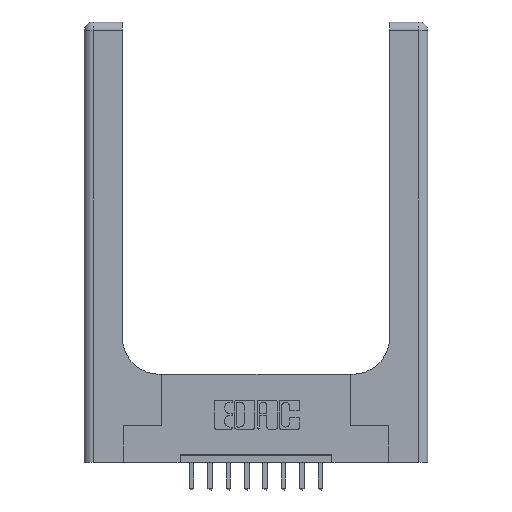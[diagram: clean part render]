
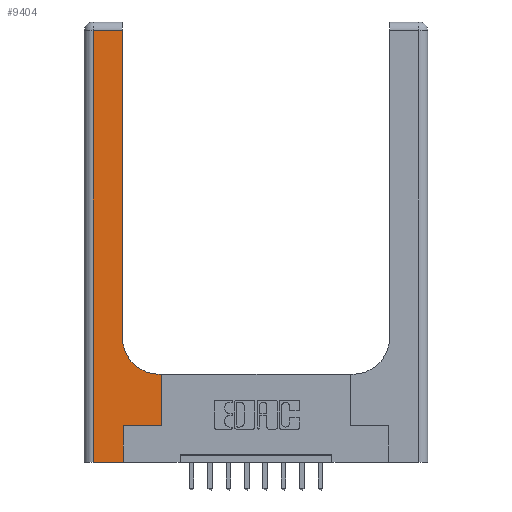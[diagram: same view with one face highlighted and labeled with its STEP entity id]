
A CAD part, top view. The second image highlights one B-rep face of the part: STEP entity #9404.
In plain terms, the highlighted planar face has unit normal (0, 0, 1).
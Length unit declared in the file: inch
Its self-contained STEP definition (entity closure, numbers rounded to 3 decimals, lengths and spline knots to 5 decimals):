
#17 = EDGE_CURVE ( 'NONE', #7598, #47, #6807, .T. ) ;
#47 = VERTEX_POINT ( 'NONE', #12666 ) ;
#351 = EDGE_LOOP ( 'NONE', ( #14441, #14775, #10858, #5102, #4295, #1513, #2029, #2494, #5639 ) ) ;
#426 = VECTOR ( 'NONE', #8383, 39.37008 ) ;
#688 = EDGE_CURVE ( 'NONE', #1045, #2866, #15166, .T. ) ;
#714 = CARTESIAN_POINT ( 'NONE',  ( 0.265, 0.25, 0.37 ) ) ;
#729 = DIRECTION ( 'NONE',  ( -1., 0., 0. ) ) ;
#1045 = VERTEX_POINT ( 'NONE', #714 ) ;
#1513 = ORIENTED_EDGE ( 'NONE', *, *, #688, .T. ) ;
#1601 = EDGE_CURVE ( 'NONE', #14572, #1045, #3699, .T. ) ;
#1659 = CARTESIAN_POINT ( 'NONE',  ( 0.06, 2.94, 0.37 ) ) ;
#1665 = VECTOR ( 'NONE', #5672, 39.37008 ) ;
#2029 = ORIENTED_EDGE ( 'NONE', *, *, #13787, .T. ) ;
#2047 = LINE ( 'NONE', #6753, #11242 ) ;
#2494 = ORIENTED_EDGE ( 'NONE', *, *, #17, .T. ) ;
#2580 = VERTEX_POINT ( 'NONE', #12955 ) ;
#2866 = VERTEX_POINT ( 'NONE', #6545 ) ;
#2950 = CARTESIAN_POINT ( 'NONE',  ( 0.265, 0., 0.37 ) ) ;
#3580 = EDGE_CURVE ( 'NONE', #2580, #14572, #5017, .T. ) ;
#3699 = LINE ( 'NONE', #5850, #426 ) ;
#4295 = ORIENTED_EDGE ( 'NONE', *, *, #1601, .T. ) ;
#4418 = DIRECTION ( 'NONE',  ( 0., 0., -1. ) ) ;
#4563 = DIRECTION ( 'NONE',  ( -1., 0., 0. ) ) ;
#4604 = VECTOR ( 'NONE', #15259, 39.37008 ) ;
#4774 = DIRECTION ( 'NONE',  ( 1., 0., 0. ) ) ;
#4850 = VERTEX_POINT ( 'NONE', #1659 ) ;
#5017 = LINE ( 'NONE', #6262, #9149 ) ;
#5102 = ORIENTED_EDGE ( 'NONE', *, *, #3580, .T. ) ;
#5385 = DIRECTION ( 'NONE',  ( 0., 1., 0. ) ) ;
#5576 = DIRECTION ( 'NONE',  ( 1., 0., 0. ) ) ;
#5639 = ORIENTED_EDGE ( 'NONE', *, *, #14768, .T. ) ;
#5672 = DIRECTION ( 'NONE',  ( 0., 1., 0. ) ) ;
#5713 = PLANE ( 'NONE',  #10213 ) ;
#5850 = CARTESIAN_POINT ( 'NONE',  ( 0.265, 0., 0.37 ) ) ;
#6116 = VECTOR ( 'NONE', #5385, 39.37008 ) ;
#6262 = CARTESIAN_POINT ( 'NONE',  ( 0., 0., 0.37 ) ) ;
#6458 = CARTESIAN_POINT ( 'NONE',  ( 0.26, 0.85, 0.37 ) ) ;
#6545 = CARTESIAN_POINT ( 'NONE',  ( 0.528, 0.25, 0.37 ) ) ;
#6553 = CARTESIAN_POINT ( 'NONE',  ( 0.26, 3., 0.37 ) ) ;
#6753 = CARTESIAN_POINT ( 'NONE',  ( 0., 2.94, 0.37 ) ) ;
#6780 = LINE ( 'NONE', #6553, #6116 ) ;
#6807 = LINE ( 'NONE', #9025, #13244 ) ;
#6991 = LINE ( 'NONE', #11694, #4604 ) ;
#7102 = CARTESIAN_POINT ( 'NONE',  ( 0.51, 0.85, 0.37 ) ) ;
#7260 = VECTOR ( 'NONE', #5576, 39.37008 ) ;
#7598 = VERTEX_POINT ( 'NONE', #15268 ) ;
#7969 = CARTESIAN_POINT ( 'NONE',  ( 0.265, 0.25, 0.37 ) ) ;
#8383 = DIRECTION ( 'NONE',  ( 0., 1., 0. ) ) ;
#9025 = CARTESIAN_POINT ( 'NONE',  ( 0.26, 0.6, 0.37 ) ) ;
#9057 = CARTESIAN_POINT ( 'NONE',  ( 0.26, 2.94, 0.37 ) ) ;
#9149 = VECTOR ( 'NONE', #12057, 39.37008 ) ;
#9404 = ADVANCED_FACE ( 'NONE', ( #15011 ), #5713, .F. ) ;
#9562 = AXIS2_PLACEMENT_3D ( 'NONE', #7102, #14204, #4774 ) ;
#10213 = AXIS2_PLACEMENT_3D ( 'NONE', #14934, #4418, #4563 ) ;
#10307 = EDGE_CURVE ( 'NONE', #12914, #4850, #2047, .T. ) ;
#10858 = ORIENTED_EDGE ( 'NONE', *, *, #13148, .T. ) ;
#11242 = VECTOR ( 'NONE', #729, 39.37008 ) ;
#11694 = CARTESIAN_POINT ( 'NONE',  ( 0.06, 3., 0.37 ) ) ;
#12057 = DIRECTION ( 'NONE',  ( 1., 0., 0. ) ) ;
#12637 = EDGE_CURVE ( 'NONE', #12993, #12914, #6780, .T. ) ;
#12666 = CARTESIAN_POINT ( 'NONE',  ( 0.51, 0.6, 0.37 ) ) ;
#12740 = DIRECTION ( 'NONE',  ( -1., 0., 0. ) ) ;
#12914 = VERTEX_POINT ( 'NONE', #9057 ) ;
#12955 = CARTESIAN_POINT ( 'NONE',  ( 0.06, 0., 0.37 ) ) ;
#12993 = VERTEX_POINT ( 'NONE', #6458 ) ;
#13148 = EDGE_CURVE ( 'NONE', #4850, #2580, #6991, .T. ) ;
#13244 = VECTOR ( 'NONE', #12740, 39.37008 ) ;
#13721 = CARTESIAN_POINT ( 'NONE',  ( 0.528, 0.25, 0.37 ) ) ;
#13787 = EDGE_CURVE ( 'NONE', #2866, #7598, #15039, .T. ) ;
#14204 = DIRECTION ( 'NONE',  ( 0., 0., -1. ) ) ;
#14441 = ORIENTED_EDGE ( 'NONE', *, *, #12637, .T. ) ;
#14501 = CIRCLE ( 'NONE', #9562, 0.25 ) ;
#14572 = VERTEX_POINT ( 'NONE', #2950 ) ;
#14768 = EDGE_CURVE ( 'NONE', #47, #12993, #14501, .T. ) ;
#14775 = ORIENTED_EDGE ( 'NONE', *, *, #10307, .T. ) ;
#14934 = CARTESIAN_POINT ( 'NONE',  ( 0., 3., 0.37 ) ) ;
#15011 = FACE_OUTER_BOUND ( 'NONE', #351, .T. ) ;
#15039 = LINE ( 'NONE', #13721, #1665 ) ;
#15166 = LINE ( 'NONE', #7969, #7260 ) ;
#15259 = DIRECTION ( 'NONE',  ( 0., -1., 0. ) ) ;
#15268 = CARTESIAN_POINT ( 'NONE',  ( 0.528, 0.6, 0.37 ) ) ;
